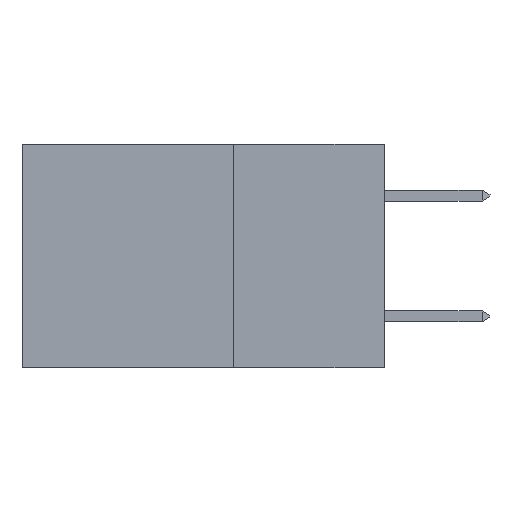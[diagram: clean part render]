
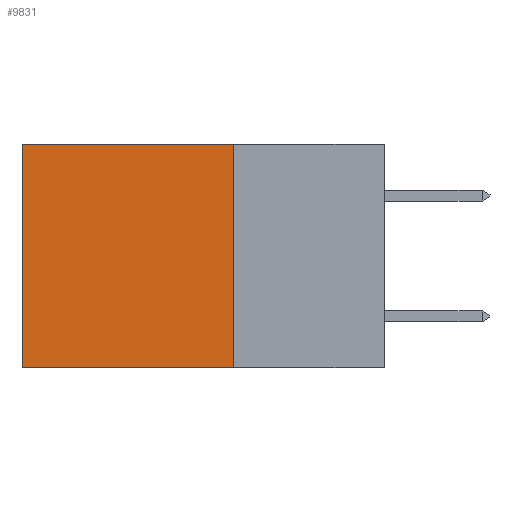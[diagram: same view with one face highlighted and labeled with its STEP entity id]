
A CAD part, left-side view. The second image highlights one B-rep face of the part: STEP entity #9831.
In plain terms, the highlighted planar face has unit normal (-1, 0, 0).
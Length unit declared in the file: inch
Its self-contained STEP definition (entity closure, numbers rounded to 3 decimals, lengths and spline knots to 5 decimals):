
#410 = AXIS2_PLACEMENT_3D ( 'NONE', #5070, #18414, #7009 ) ;
#1435 = ORIENTED_EDGE ( 'NONE', *, *, #6070, .T. ) ;
#1851 = VECTOR ( 'NONE', #23671, 39.37008 ) ;
#2425 = LINE ( 'NONE', #14324, #1851 ) ;
#3008 = EDGE_CURVE ( 'NONE', #12869, #6450, #19894, .T. ) ;
#3455 = CARTESIAN_POINT ( 'NONE',  ( 0.2875, 0.25, 0. ) ) ;
#3581 = VERTEX_POINT ( 'NONE', #10799 ) ;
#4697 = EDGE_CURVE ( 'NONE', #3581, #11974, #12117, .T. ) ;
#5070 = CARTESIAN_POINT ( 'NONE',  ( 0.2875, 0.25, 0. ) ) ;
#5258 = VECTOR ( 'NONE', #21946, 39.37008 ) ;
#5790 = CARTESIAN_POINT ( 'NONE',  ( 0.2875, 0.25, 0. ) ) ;
#6070 = EDGE_CURVE ( 'NONE', #6450, #11974, #2425, .T. ) ;
#6450 = VERTEX_POINT ( 'NONE', #22907 ) ;
#7009 = DIRECTION ( 'NONE',  ( 0., 0., -1. ) ) ;
#7342 = CARTESIAN_POINT ( 'NONE',  ( 0.2875, 0.6, -0.37 ) ) ;
#8678 = CARTESIAN_POINT ( 'NONE',  ( 0.2875, 0.25, 0. ) ) ;
#9760 = LINE ( 'NONE', #8678, #5258 ) ;
#9831 = ADVANCED_FACE ( 'NONE', ( #22574 ), #20230, .F. ) ;
#10343 = CARTESIAN_POINT ( 'NONE',  ( 0.2875, 0.25, -0.37 ) ) ;
#10799 = CARTESIAN_POINT ( 'NONE',  ( 0.2875, 0.25, -0.37 ) ) ;
#11974 = VERTEX_POINT ( 'NONE', #7342 ) ;
#12117 = LINE ( 'NONE', #10343, #17153 ) ;
#12351 = EDGE_LOOP ( 'NONE', ( #1435, #17907, #14687, #19174 ) ) ;
#12869 = VERTEX_POINT ( 'NONE', #5790 ) ;
#13125 = DIRECTION ( 'NONE',  ( 0., 1., 0. ) ) ;
#14324 = CARTESIAN_POINT ( 'NONE',  ( 0.2875, 0.6, 0. ) ) ;
#14687 = ORIENTED_EDGE ( 'NONE', *, *, #19612, .F. ) ;
#15999 = DIRECTION ( 'NONE',  ( 0., 1., 0. ) ) ;
#17153 = VECTOR ( 'NONE', #15999, 39.37008 ) ;
#17907 = ORIENTED_EDGE ( 'NONE', *, *, #4697, .F. ) ;
#18414 = DIRECTION ( 'NONE',  ( 1., 0., 0. ) ) ;
#19174 = ORIENTED_EDGE ( 'NONE', *, *, #3008, .T. ) ;
#19612 = EDGE_CURVE ( 'NONE', #12869, #3581, #9760, .T. ) ;
#19894 = LINE ( 'NONE', #3455, #24328 ) ;
#20230 = PLANE ( 'NONE',  #410 ) ;
#21946 = DIRECTION ( 'NONE',  ( 0., 0., -1. ) ) ;
#22574 = FACE_OUTER_BOUND ( 'NONE', #12351, .T. ) ;
#22907 = CARTESIAN_POINT ( 'NONE',  ( 0.2875, 0.6, 0. ) ) ;
#23671 = DIRECTION ( 'NONE',  ( 0., 0., -1. ) ) ;
#24328 = VECTOR ( 'NONE', #13125, 39.37008 ) ;
